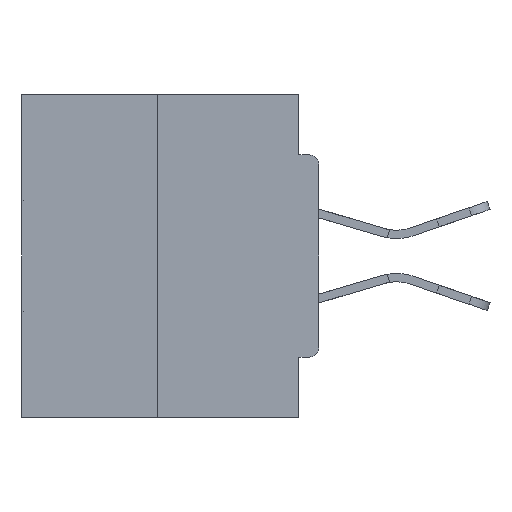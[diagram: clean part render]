
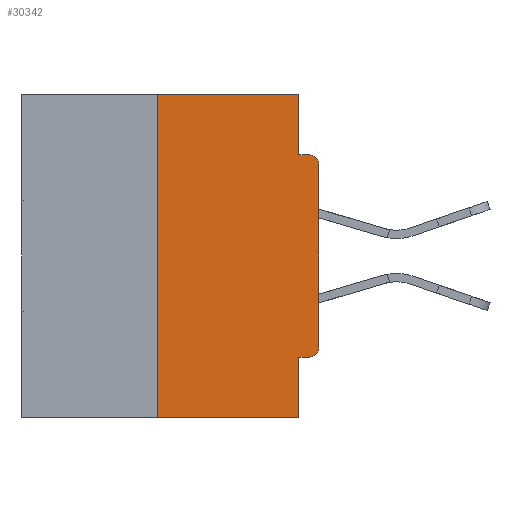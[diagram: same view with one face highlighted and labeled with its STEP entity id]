
A CAD part, left-side view. The second image highlights one B-rep face of the part: STEP entity #30342.
In plain terms, the highlighted planar face has unit normal (-1, 0, 0).
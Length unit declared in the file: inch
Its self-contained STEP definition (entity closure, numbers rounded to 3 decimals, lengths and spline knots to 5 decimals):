
#1117 = LINE ( 'NONE', #35685, #6436 ) ;
#1589 = EDGE_CURVE ( 'NONE', #6274, #26591, #32110, .T. ) ;
#1901 = CARTESIAN_POINT ( 'NONE',  ( 0., 0.031, -0.5 ) ) ;
#2104 = CARTESIAN_POINT ( 'NONE',  ( 0., 0.46, 0. ) ) ;
#2529 = EDGE_LOOP ( 'NONE', ( #18467, #17776, #28524, #33600, #23812, #28003, #31809, #19393, #39239, #10368 ) ) ;
#3012 = DIRECTION ( 'NONE',  ( -1., 0., 0. ) ) ;
#3483 = VECTOR ( 'NONE', #36699, 39.37008 ) ;
#3753 = EDGE_CURVE ( 'NONE', #4153, #6676, #11443, .T. ) ;
#3949 = LINE ( 'NONE', #16376, #24493 ) ;
#4153 = VERTEX_POINT ( 'NONE', #21786 ) ;
#4700 = DIRECTION ( 'NONE',  ( -1., 0., 0. ) ) ;
#5207 = VERTEX_POINT ( 'NONE', #37816 ) ;
#5488 = CARTESIAN_POINT ( 'NONE',  ( 0., 0.031, 0. ) ) ;
#5518 = VECTOR ( 'NONE', #17997, 39.37008 ) ;
#5652 = EDGE_CURVE ( 'NONE', #34793, #4153, #3949, .T. ) ;
#6274 = VERTEX_POINT ( 'NONE', #9384 ) ;
#6436 = VECTOR ( 'NONE', #14177, 39.37008 ) ;
#6546 = AXIS2_PLACEMENT_3D ( 'NONE', #13753, #4700, #26716 ) ;
#6676 = VERTEX_POINT ( 'NONE', #36958 ) ;
#7496 = VERTEX_POINT ( 'NONE', #5488 ) ;
#7648 = LINE ( 'NONE', #37874, #15480 ) ;
#8221 = PLANE ( 'NONE',  #20269 ) ;
#9384 = CARTESIAN_POINT ( 'NONE',  ( 0., 0.031, -0.4065 ) ) ;
#9649 = DIRECTION ( 'NONE',  ( 0., -1., 0. ) ) ;
#10222 = EDGE_CURVE ( 'NONE', #10816, #6676, #38381, .T. ) ;
#10368 = ORIENTED_EDGE ( 'NONE', *, *, #16848, .F. ) ;
#10543 = CARTESIAN_POINT ( 'NONE',  ( 0., 0.25, 0. ) ) ;
#10816 = VERTEX_POINT ( 'NONE', #29807 ) ;
#11443 = CIRCLE ( 'NONE', #18489, 0.015 ) ;
#11627 = CARTESIAN_POINT ( 'NONE',  ( 0., 0.031, 0. ) ) ;
#11671 = VECTOR ( 'NONE', #28818, 39.37008 ) ;
#12560 = CARTESIAN_POINT ( 'NONE',  ( 0., 0.015, -0.1085 ) ) ;
#13035 = CARTESIAN_POINT ( 'NONE',  ( 0., 0., -0.3915 ) ) ;
#13114 = EDGE_CURVE ( 'NONE', #33643, #7496, #14580, .T. ) ;
#13753 = CARTESIAN_POINT ( 'NONE',  ( 0., 0.015, -0.3915 ) ) ;
#14177 = DIRECTION ( 'NONE',  ( 0., 1., 0. ) ) ;
#14580 = LINE ( 'NONE', #23302, #11671 ) ;
#14672 = LINE ( 'NONE', #20694, #22031 ) ;
#15480 = VECTOR ( 'NONE', #9649, 39.37008 ) ;
#15787 = CARTESIAN_POINT ( 'NONE',  ( 0., 0.25, -0.5 ) ) ;
#16376 = CARTESIAN_POINT ( 'NONE',  ( 0., 0., 0. ) ) ;
#16848 = EDGE_CURVE ( 'NONE', #7496, #10816, #36294, .T. ) ;
#17645 = DIRECTION ( 'NONE',  ( 0., 0., -1. ) ) ;
#17776 = ORIENTED_EDGE ( 'NONE', *, *, #29541, .F. ) ;
#17924 = EDGE_CURVE ( 'NONE', #5207, #34793, #27360, .T. ) ;
#17997 = DIRECTION ( 'NONE',  ( 0., -1., 0. ) ) ;
#18467 = ORIENTED_EDGE ( 'NONE', *, *, #13114, .F. ) ;
#18489 = AXIS2_PLACEMENT_3D ( 'NONE', #12560, #3012, #34447 ) ;
#18874 = VECTOR ( 'NONE', #23906, 39.37008 ) ;
#18986 = DIRECTION ( 'NONE',  ( 0., 0., 1. ) ) ;
#19393 = ORIENTED_EDGE ( 'NONE', *, *, #3753, .T. ) ;
#20269 = AXIS2_PLACEMENT_3D ( 'NONE', #2104, #30395, #17645 ) ;
#20694 = CARTESIAN_POINT ( 'NONE',  ( 0., 0.25, 0. ) ) ;
#21786 = CARTESIAN_POINT ( 'NONE',  ( 0., 0., -0.1085 ) ) ;
#22031 = VECTOR ( 'NONE', #33541, 39.37008 ) ;
#23302 = CARTESIAN_POINT ( 'NONE',  ( 0., 0.46, 0. ) ) ;
#23479 = EDGE_CURVE ( 'NONE', #29965, #26591, #7648, .T. ) ;
#23812 = ORIENTED_EDGE ( 'NONE', *, *, #26406, .F. ) ;
#23906 = DIRECTION ( 'NONE',  ( 0., 0., -1. ) ) ;
#24493 = VECTOR ( 'NONE', #18986, 39.37008 ) ;
#26406 = EDGE_CURVE ( 'NONE', #5207, #6274, #1117, .T. ) ;
#26591 = VERTEX_POINT ( 'NONE', #40374 ) ;
#26716 = DIRECTION ( 'NONE',  ( 0., 0., -1. ) ) ;
#27360 = CIRCLE ( 'NONE', #6546, 0.015 ) ;
#28003 = ORIENTED_EDGE ( 'NONE', *, *, #17924, .T. ) ;
#28524 = ORIENTED_EDGE ( 'NONE', *, *, #23479, .T. ) ;
#28818 = DIRECTION ( 'NONE',  ( 0., -1., 0. ) ) ;
#29541 = EDGE_CURVE ( 'NONE', #29965, #33643, #14672, .T. ) ;
#29807 = CARTESIAN_POINT ( 'NONE',  ( 0., 0.031, -0.0935 ) ) ;
#29965 = VERTEX_POINT ( 'NONE', #15787 ) ;
#30342 = ADVANCED_FACE ( 'NONE', ( #32246 ), #8221, .F. ) ;
#30395 = DIRECTION ( 'NONE',  ( 1., 0., 0. ) ) ;
#31809 = ORIENTED_EDGE ( 'NONE', *, *, #5652, .T. ) ;
#32110 = LINE ( 'NONE', #1901, #18874 ) ;
#32246 = FACE_OUTER_BOUND ( 'NONE', #2529, .T. ) ;
#33541 = DIRECTION ( 'NONE',  ( 0., 0., 1. ) ) ;
#33600 = ORIENTED_EDGE ( 'NONE', *, *, #1589, .F. ) ;
#33643 = VERTEX_POINT ( 'NONE', #10543 ) ;
#34447 = DIRECTION ( 'NONE',  ( 0., 0., -1. ) ) ;
#34793 = VERTEX_POINT ( 'NONE', #13035 ) ;
#35685 = CARTESIAN_POINT ( 'NONE',  ( 0., 0., -0.4065 ) ) ;
#36294 = LINE ( 'NONE', #11627, #3483 ) ;
#36699 = DIRECTION ( 'NONE',  ( 0., 0., -1. ) ) ;
#36958 = CARTESIAN_POINT ( 'NONE',  ( 0., 0.015, -0.0935 ) ) ;
#37064 = CARTESIAN_POINT ( 'NONE',  ( 0., 0., -0.0935 ) ) ;
#37816 = CARTESIAN_POINT ( 'NONE',  ( 0., 0.015, -0.4065 ) ) ;
#37874 = CARTESIAN_POINT ( 'NONE',  ( 0., 0.46, -0.5 ) ) ;
#38381 = LINE ( 'NONE', #37064, #5518 ) ;
#39239 = ORIENTED_EDGE ( 'NONE', *, *, #10222, .F. ) ;
#40374 = CARTESIAN_POINT ( 'NONE',  ( 0., 0.031, -0.5 ) ) ;
